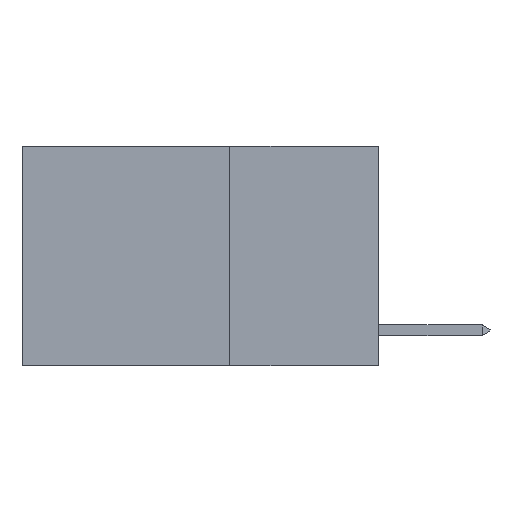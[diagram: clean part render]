
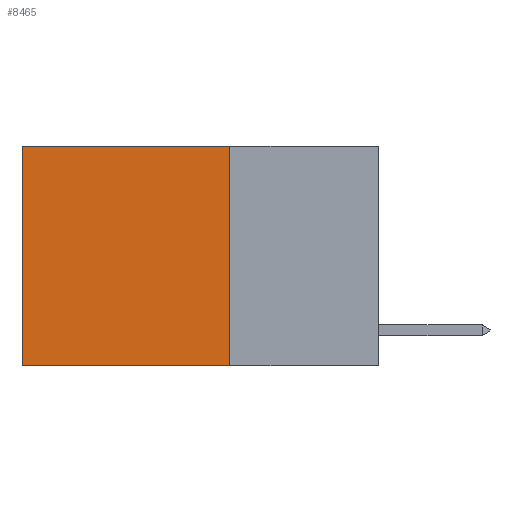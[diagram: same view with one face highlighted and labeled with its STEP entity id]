
A CAD part, left-side view. The second image highlights one B-rep face of the part: STEP entity #8465.
In plain terms, the highlighted planar face has unit normal (-1, 0, 0).
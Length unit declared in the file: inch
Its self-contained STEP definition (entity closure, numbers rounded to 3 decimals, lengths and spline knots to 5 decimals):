
#67 = CARTESIAN_POINT ( 'NONE',  ( 0.2625, 0.25, -0.37 ) ) ;
#202 = VECTOR ( 'NONE', #934, 39.37008 ) ;
#430 = CARTESIAN_POINT ( 'NONE',  ( 0.2625, 0.25, 0. ) ) ;
#437 = CARTESIAN_POINT ( 'NONE',  ( 0.2625, 0.25, 0. ) ) ;
#926 = EDGE_CURVE ( 'NONE', #5315, #10666, #6573, .T. ) ;
#934 = DIRECTION ( 'NONE',  ( 0., 1., 0. ) ) ;
#1573 = DIRECTION ( 'NONE',  ( 0., 0., -1. ) ) ;
#1580 = DIRECTION ( 'NONE',  ( 0., 0., -1. ) ) ;
#2335 = DIRECTION ( 'NONE',  ( 0., 1., 0. ) ) ;
#3265 = CARTESIAN_POINT ( 'NONE',  ( 0.2625, 0.25, -0.37 ) ) ;
#4084 = ORIENTED_EDGE ( 'NONE', *, *, #11989, .T. ) ;
#4658 = CARTESIAN_POINT ( 'NONE',  ( 0.2625, 0.6, -0.37 ) ) ;
#4901 = PLANE ( 'NONE',  #8127 ) ;
#5315 = VERTEX_POINT ( 'NONE', #6388 ) ;
#5522 = DIRECTION ( 'NONE',  ( 0., 0., -1. ) ) ;
#5656 = EDGE_LOOP ( 'NONE', ( #4084, #11584, #8316, #11119 ) ) ;
#6189 = LINE ( 'NONE', #6535, #202 ) ;
#6229 = VECTOR ( 'NONE', #1580, 39.37008 ) ;
#6388 = CARTESIAN_POINT ( 'NONE',  ( 0.2625, 0.25, 0. ) ) ;
#6535 = CARTESIAN_POINT ( 'NONE',  ( 0.2625, 0.25, 0. ) ) ;
#6573 = LINE ( 'NONE', #437, #6229 ) ;
#7014 = VERTEX_POINT ( 'NONE', #4658 ) ;
#7821 = LINE ( 'NONE', #10111, #10489 ) ;
#8127 = AXIS2_PLACEMENT_3D ( 'NONE', #430, #8373, #1573 ) ;
#8316 = ORIENTED_EDGE ( 'NONE', *, *, #926, .F. ) ;
#8373 = DIRECTION ( 'NONE',  ( 1., 0., 0. ) ) ;
#8465 = ADVANCED_FACE ( 'NONE', ( #12936 ), #4901, .F. ) ;
#8904 = VERTEX_POINT ( 'NONE', #13849 ) ;
#10084 = LINE ( 'NONE', #67, #13124 ) ;
#10111 = CARTESIAN_POINT ( 'NONE',  ( 0.2625, 0.6, 0. ) ) ;
#10489 = VECTOR ( 'NONE', #5522, 39.37008 ) ;
#10666 = VERTEX_POINT ( 'NONE', #3265 ) ;
#11119 = ORIENTED_EDGE ( 'NONE', *, *, #11904, .T. ) ;
#11584 = ORIENTED_EDGE ( 'NONE', *, *, #14540, .F. ) ;
#11904 = EDGE_CURVE ( 'NONE', #5315, #8904, #6189, .T. ) ;
#11989 = EDGE_CURVE ( 'NONE', #8904, #7014, #7821, .T. ) ;
#12936 = FACE_OUTER_BOUND ( 'NONE', #5656, .T. ) ;
#13124 = VECTOR ( 'NONE', #2335, 39.37008 ) ;
#13849 = CARTESIAN_POINT ( 'NONE',  ( 0.2625, 0.6, 0. ) ) ;
#14540 = EDGE_CURVE ( 'NONE', #10666, #7014, #10084, .T. ) ;
